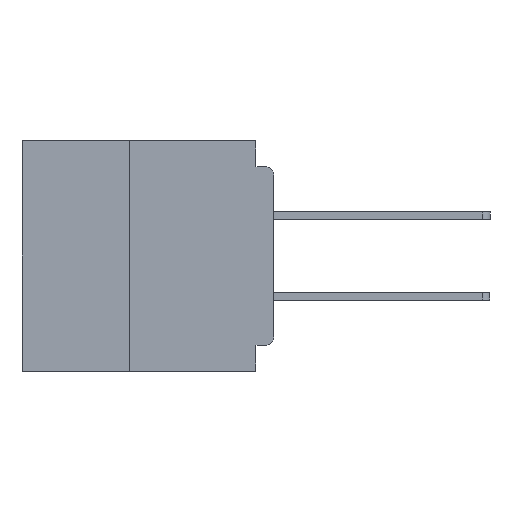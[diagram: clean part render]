
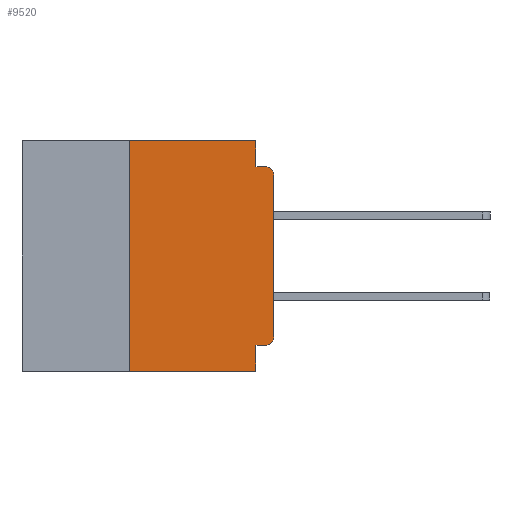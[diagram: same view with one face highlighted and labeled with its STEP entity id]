
A CAD part, left-side view. The second image highlights one B-rep face of the part: STEP entity #9520.
In plain terms, the highlighted planar face has unit normal (-1, 0, 0).
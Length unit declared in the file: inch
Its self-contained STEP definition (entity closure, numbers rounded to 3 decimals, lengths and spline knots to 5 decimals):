
#368 = ORIENTED_EDGE ( 'NONE', *, *, #15816, .F. ) ;
#882 = VECTOR ( 'NONE', #14406, 39.37008 ) ;
#1269 = ORIENTED_EDGE ( 'NONE', *, *, #16531, .F. ) ;
#1642 = DIRECTION ( 'NONE',  ( 0., 0., -1. ) ) ;
#2004 = EDGE_CURVE ( 'NONE', #20602, #12766, #5319, .T. ) ;
#2219 = CARTESIAN_POINT ( 'NONE',  ( 0., 0.015, -0.06 ) ) ;
#2440 = DIRECTION ( 'NONE',  ( 0., -1., 0. ) ) ;
#2764 = EDGE_CURVE ( 'NONE', #7003, #39377, #33873, .T. ) ;
#3082 = VERTEX_POINT ( 'NONE', #3420 ) ;
#3100 = CIRCLE ( 'NONE', #15351, 0.015 ) ;
#3229 = CARTESIAN_POINT ( 'NONE',  ( 0., 0., -0.045 ) ) ;
#3396 = EDGE_CURVE ( 'NONE', #8319, #12766, #3100, .T. ) ;
#3420 = CARTESIAN_POINT ( 'NONE',  ( 0., 0.25, 0. ) ) ;
#3516 = DIRECTION ( 'NONE',  ( 0., 1., 0. ) ) ;
#3900 = CARTESIAN_POINT ( 'NONE',  ( 0., 0.437, 0. ) ) ;
#4035 = LINE ( 'NONE', #28318, #23458 ) ;
#5319 = LINE ( 'NONE', #3229, #13607 ) ;
#5346 = DIRECTION ( 'NONE',  ( 0., 0., -1. ) ) ;
#6135 = EDGE_CURVE ( 'NONE', #7753, #39377, #14820, .T. ) ;
#7003 = VERTEX_POINT ( 'NONE', #16309 ) ;
#7085 = VECTOR ( 'NONE', #1642, 39.37008 ) ;
#7294 = CARTESIAN_POINT ( 'NONE',  ( 0., 0.031, -0.4 ) ) ;
#7435 = LINE ( 'NONE', #12491, #31233 ) ;
#7589 = CARTESIAN_POINT ( 'NONE',  ( 0., 0.015, -0.34 ) ) ;
#7753 = VERTEX_POINT ( 'NONE', #21829 ) ;
#8319 = VERTEX_POINT ( 'NONE', #36952 ) ;
#8460 = CARTESIAN_POINT ( 'NONE',  ( 0., 0.031, 0. ) ) ;
#9520 = ADVANCED_FACE ( 'NONE', ( #39700 ), #18613, .F. ) ;
#9648 = CARTESIAN_POINT ( 'NONE',  ( 0., 0., -0.355 ) ) ;
#9739 = DIRECTION ( 'NONE',  ( 0., 0., 1. ) ) ;
#9842 = AXIS2_PLACEMENT_3D ( 'NONE', #34023, #20277, #21697 ) ;
#10270 = VERTEX_POINT ( 'NONE', #8460 ) ;
#10674 = VERTEX_POINT ( 'NONE', #29879 ) ;
#10695 = ORIENTED_EDGE ( 'NONE', *, *, #6135, .T. ) ;
#10757 = DIRECTION ( 'NONE',  ( 0., 0., -1. ) ) ;
#12491 = CARTESIAN_POINT ( 'NONE',  ( 0., 0.25, -0.4 ) ) ;
#12766 = VERTEX_POINT ( 'NONE', #27406 ) ;
#13271 = DIRECTION ( 'NONE',  ( 0., -1., 0. ) ) ;
#13513 = EDGE_LOOP ( 'NONE', ( #17860, #21969, #23814, #34630, #1269, #368, #10695, #36961, #39722, #34238 ) ) ;
#13607 = VECTOR ( 'NONE', #2440, 39.37008 ) ;
#14264 = EDGE_CURVE ( 'NONE', #10270, #20602, #15376, .T. ) ;
#14406 = DIRECTION ( 'NONE',  ( 0., 0., -1. ) ) ;
#14768 = CARTESIAN_POINT ( 'NONE',  ( 0., 0.031, -0.4 ) ) ;
#14820 = LINE ( 'NONE', #21378, #37577 ) ;
#15351 = AXIS2_PLACEMENT_3D ( 'NONE', #2219, #23935, #5346 ) ;
#15376 = LINE ( 'NONE', #29326, #7085 ) ;
#15816 = EDGE_CURVE ( 'NONE', #7753, #3082, #7435, .T. ) ;
#15878 = EDGE_CURVE ( 'NONE', #10674, #7003, #36548, .T. ) ;
#16309 = CARTESIAN_POINT ( 'NONE',  ( 0., 0.031, -0.355 ) ) ;
#16531 = EDGE_CURVE ( 'NONE', #3082, #10270, #28773, .T. ) ;
#17198 = CARTESIAN_POINT ( 'NONE',  ( 0., 0., -0.34 ) ) ;
#17860 = ORIENTED_EDGE ( 'NONE', *, *, #18418, .T. ) ;
#18418 = EDGE_CURVE ( 'NONE', #30362, #8319, #4035, .T. ) ;
#18613 = PLANE ( 'NONE',  #9842 ) ;
#18831 = CARTESIAN_POINT ( 'NONE',  ( 0., 0.031, -0.045 ) ) ;
#20277 = DIRECTION ( 'NONE',  ( 1., 0., 0. ) ) ;
#20542 = VECTOR ( 'NONE', #13271, 39.37008 ) ;
#20602 = VERTEX_POINT ( 'NONE', #18831 ) ;
#21378 = CARTESIAN_POINT ( 'NONE',  ( 0., 0.437, -0.4 ) ) ;
#21697 = DIRECTION ( 'NONE',  ( 0., 0., -1. ) ) ;
#21829 = CARTESIAN_POINT ( 'NONE',  ( 0., 0.25, -0.4 ) ) ;
#21969 = ORIENTED_EDGE ( 'NONE', *, *, #3396, .T. ) ;
#23458 = VECTOR ( 'NONE', #9739, 39.37008 ) ;
#23639 = CIRCLE ( 'NONE', #28531, 0.015 ) ;
#23814 = ORIENTED_EDGE ( 'NONE', *, *, #2004, .F. ) ;
#23935 = DIRECTION ( 'NONE',  ( -1., 0., 0. ) ) ;
#27406 = CARTESIAN_POINT ( 'NONE',  ( 0., 0.015, -0.045 ) ) ;
#27477 = DIRECTION ( 'NONE',  ( 0., -1., 0. ) ) ;
#28318 = CARTESIAN_POINT ( 'NONE',  ( 0., 0., 0. ) ) ;
#28335 = VECTOR ( 'NONE', #3516, 39.37008 ) ;
#28531 = AXIS2_PLACEMENT_3D ( 'NONE', #7589, #29332, #10757 ) ;
#28773 = LINE ( 'NONE', #3900, #20542 ) ;
#29326 = CARTESIAN_POINT ( 'NONE',  ( 0., 0.031, 0. ) ) ;
#29332 = DIRECTION ( 'NONE',  ( -1., 0., 0. ) ) ;
#29879 = CARTESIAN_POINT ( 'NONE',  ( 0., 0.015, -0.355 ) ) ;
#30362 = VERTEX_POINT ( 'NONE', #17198 ) ;
#31054 = DIRECTION ( 'NONE',  ( 0., 0., 1. ) ) ;
#31233 = VECTOR ( 'NONE', #31054, 39.37008 ) ;
#33873 = LINE ( 'NONE', #14768, #882 ) ;
#34023 = CARTESIAN_POINT ( 'NONE',  ( 0., 0.437, 0. ) ) ;
#34238 = ORIENTED_EDGE ( 'NONE', *, *, #38157, .T. ) ;
#34630 = ORIENTED_EDGE ( 'NONE', *, *, #14264, .F. ) ;
#36548 = LINE ( 'NONE', #9648, #28335 ) ;
#36952 = CARTESIAN_POINT ( 'NONE',  ( 0., 0., -0.06 ) ) ;
#36961 = ORIENTED_EDGE ( 'NONE', *, *, #2764, .F. ) ;
#37577 = VECTOR ( 'NONE', #27477, 39.37008 ) ;
#38157 = EDGE_CURVE ( 'NONE', #10674, #30362, #23639, .T. ) ;
#39377 = VERTEX_POINT ( 'NONE', #7294 ) ;
#39700 = FACE_OUTER_BOUND ( 'NONE', #13513, .T. ) ;
#39722 = ORIENTED_EDGE ( 'NONE', *, *, #15878, .F. ) ;
